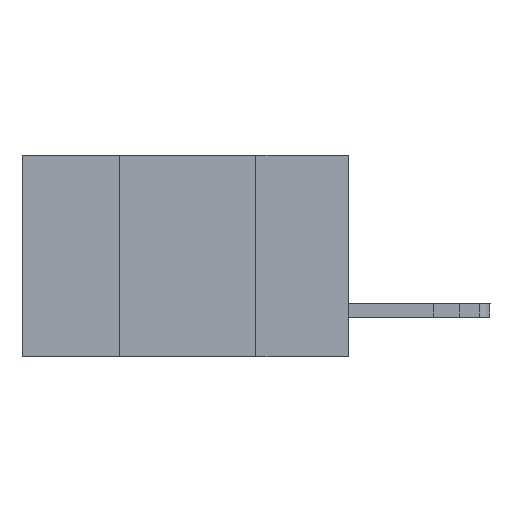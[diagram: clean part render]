
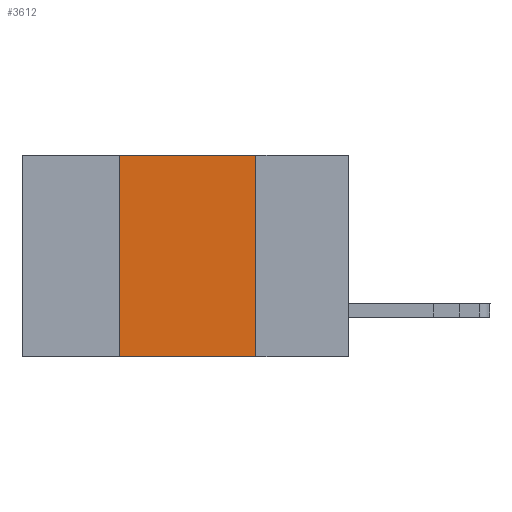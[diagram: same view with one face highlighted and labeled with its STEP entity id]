
A CAD part, left-side view. The second image highlights one B-rep face of the part: STEP entity #3612.
In plain terms, the highlighted planar face has unit normal (-1, 0, 0).
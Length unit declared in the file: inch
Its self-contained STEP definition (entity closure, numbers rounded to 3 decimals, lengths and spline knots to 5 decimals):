
#48 = ORIENTED_EDGE ( 'NONE', *, *, #4612, .T. ) ;
#655 = EDGE_CURVE ( 'NONE', #796, #8666, #12435, .T. ) ;
#780 = LINE ( 'NONE', #10008, #10414 ) ;
#796 = VERTEX_POINT ( 'NONE', #8957 ) ;
#1632 = CARTESIAN_POINT ( 'NONE',  ( 0., 0.42, -0.37 ) ) ;
#1760 = DIRECTION ( 'NONE',  ( 0., -1., 0. ) ) ;
#1792 = CARTESIAN_POINT ( 'NONE',  ( 0., 0.42, 0. ) ) ;
#1941 = CARTESIAN_POINT ( 'NONE',  ( 0., 0.42, -0.37 ) ) ;
#1985 = EDGE_CURVE ( 'NONE', #7609, #796, #10187, .T. ) ;
#2093 = DIRECTION ( 'NONE',  ( 0., 0., 1. ) ) ;
#2188 = CARTESIAN_POINT ( 'NONE',  ( 0., 0.17, -0.37 ) ) ;
#2382 = CARTESIAN_POINT ( 'NONE',  ( 0., 0.17, -0.37 ) ) ;
#2621 = DIRECTION ( 'NONE',  ( 0., 0., -1. ) ) ;
#3068 = CARTESIAN_POINT ( 'NONE',  ( 0., 0.6, 0. ) ) ;
#3249 = DIRECTION ( 'NONE',  ( 0., 0., -1. ) ) ;
#3265 = DIRECTION ( 'NONE',  ( 1., 0., 0. ) ) ;
#3551 = PLANE ( 'NONE',  #4209 ) ;
#3612 = ADVANCED_FACE ( 'NONE', ( #11948 ), #3551, .F. ) ;
#3993 = EDGE_CURVE ( 'NONE', #8843, #7609, #8030, .T. ) ;
#4209 = AXIS2_PLACEMENT_3D ( 'NONE', #3068, #3265, #3249 ) ;
#4612 = EDGE_CURVE ( 'NONE', #8843, #8666, #780, .T. ) ;
#5654 = EDGE_LOOP ( 'NONE', ( #7174, #9739, #7475, #48 ) ) ;
#7174 = ORIENTED_EDGE ( 'NONE', *, *, #655, .F. ) ;
#7322 = VECTOR ( 'NONE', #1760, 39.37008 ) ;
#7358 = VECTOR ( 'NONE', #2621, 39.37008 ) ;
#7475 = ORIENTED_EDGE ( 'NONE', *, *, #3993, .F. ) ;
#7609 = VERTEX_POINT ( 'NONE', #1792 ) ;
#7724 = VECTOR ( 'NONE', #2093, 39.37008 ) ;
#8030 = LINE ( 'NONE', #1941, #7724 ) ;
#8666 = VERTEX_POINT ( 'NONE', #2382 ) ;
#8843 = VERTEX_POINT ( 'NONE', #1632 ) ;
#8957 = CARTESIAN_POINT ( 'NONE',  ( 0., 0.17, 0. ) ) ;
#9739 = ORIENTED_EDGE ( 'NONE', *, *, #1985, .F. ) ;
#10008 = CARTESIAN_POINT ( 'NONE',  ( 0., 0.6, -0.37 ) ) ;
#10187 = LINE ( 'NONE', #12078, #7322 ) ;
#10414 = VECTOR ( 'NONE', #12079, 39.37008 ) ;
#11948 = FACE_OUTER_BOUND ( 'NONE', #5654, .T. ) ;
#12078 = CARTESIAN_POINT ( 'NONE',  ( 0., 0.6, 0. ) ) ;
#12079 = DIRECTION ( 'NONE',  ( 0., -1., 0. ) ) ;
#12435 = LINE ( 'NONE', #2188, #7358 ) ;
